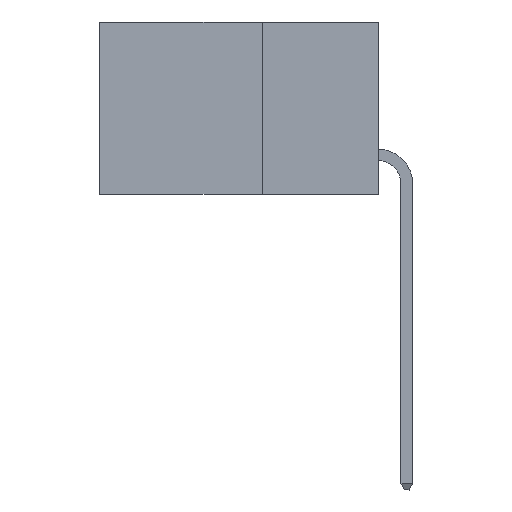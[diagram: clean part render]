
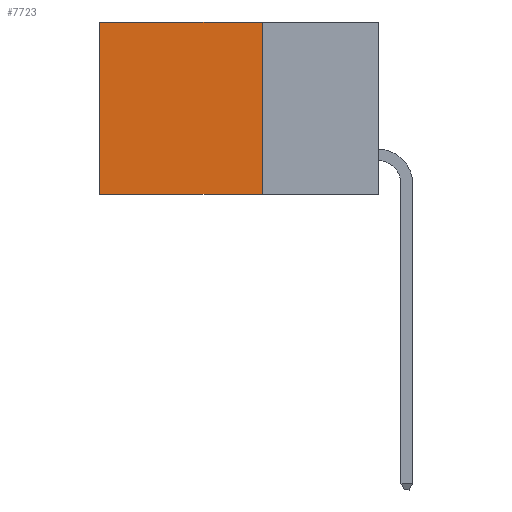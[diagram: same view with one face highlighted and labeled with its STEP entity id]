
A CAD part, left-side view. The second image highlights one B-rep face of the part: STEP entity #7723.
In plain terms, the highlighted planar face has unit normal (-1, 0, 0).
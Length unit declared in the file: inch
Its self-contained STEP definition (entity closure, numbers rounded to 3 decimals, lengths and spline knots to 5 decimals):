
#1547 = PLANE ( 'NONE',  #17949 ) ;
#1715 = VERTEX_POINT ( 'NONE', #7230 ) ;
#2119 = DIRECTION ( 'NONE',  ( 0., 0., -1. ) ) ;
#2661 = EDGE_CURVE ( 'NONE', #3821, #1715, #15868, .T. ) ;
#2883 = FACE_OUTER_BOUND ( 'NONE', #20811, .T. ) ;
#3042 = ORIENTED_EDGE ( 'NONE', *, *, #2661, .T. ) ;
#3354 = CARTESIAN_POINT ( 'NONE',  ( 0.298, 0.25, 0. ) ) ;
#3821 = VERTEX_POINT ( 'NONE', #21715 ) ;
#4376 = VERTEX_POINT ( 'NONE', #21604 ) ;
#5085 = DIRECTION ( 'NONE',  ( 1., 0., 0. ) ) ;
#5947 = VECTOR ( 'NONE', #14464, 39.37008 ) ;
#6049 = EDGE_CURVE ( 'NONE', #9122, #4376, #19438, .T. ) ;
#6178 = VECTOR ( 'NONE', #2119, 39.37008 ) ;
#6713 = LINE ( 'NONE', #17418, #6178 ) ;
#6860 = VECTOR ( 'NONE', #15695, 39.37008 ) ;
#7230 = CARTESIAN_POINT ( 'NONE',  ( 0.298, 0.6, 0. ) ) ;
#7564 = ORIENTED_EDGE ( 'NONE', *, *, #6049, .F. ) ;
#7723 = ADVANCED_FACE ( 'NONE', ( #2883 ), #1547, .F. ) ;
#8510 = CARTESIAN_POINT ( 'NONE',  ( 0.298, 0.25, -0.37 ) ) ;
#9122 = VERTEX_POINT ( 'NONE', #8510 ) ;
#10770 = ORIENTED_EDGE ( 'NONE', *, *, #20663, .F. ) ;
#11560 = VECTOR ( 'NONE', #13045, 39.37008 ) ;
#13045 = DIRECTION ( 'NONE',  ( 0., 0., -1. ) ) ;
#13277 = EDGE_CURVE ( 'NONE', #1715, #4376, #20488, .T. ) ;
#13557 = CARTESIAN_POINT ( 'NONE',  ( 0.298, 0.25, 0. ) ) ;
#14395 = CARTESIAN_POINT ( 'NONE',  ( 0.298, 0.25, -0.37 ) ) ;
#14464 = DIRECTION ( 'NONE',  ( 0., 1., 0. ) ) ;
#15695 = DIRECTION ( 'NONE',  ( 0., 1., 0. ) ) ;
#15868 = LINE ( 'NONE', #13557, #6860 ) ;
#16719 = ORIENTED_EDGE ( 'NONE', *, *, #13277, .T. ) ;
#16932 = DIRECTION ( 'NONE',  ( 0., 0., -1. ) ) ;
#17418 = CARTESIAN_POINT ( 'NONE',  ( 0.298, 0.25, 0. ) ) ;
#17949 = AXIS2_PLACEMENT_3D ( 'NONE', #3354, #5085, #16932 ) ;
#18050 = CARTESIAN_POINT ( 'NONE',  ( 0.298, 0.6, 0. ) ) ;
#19438 = LINE ( 'NONE', #14395, #5947 ) ;
#20488 = LINE ( 'NONE', #18050, #11560 ) ;
#20663 = EDGE_CURVE ( 'NONE', #3821, #9122, #6713, .T. ) ;
#20811 = EDGE_LOOP ( 'NONE', ( #16719, #7564, #10770, #3042 ) ) ;
#21604 = CARTESIAN_POINT ( 'NONE',  ( 0.298, 0.6, -0.37 ) ) ;
#21715 = CARTESIAN_POINT ( 'NONE',  ( 0.298, 0.25, 0. ) ) ;
